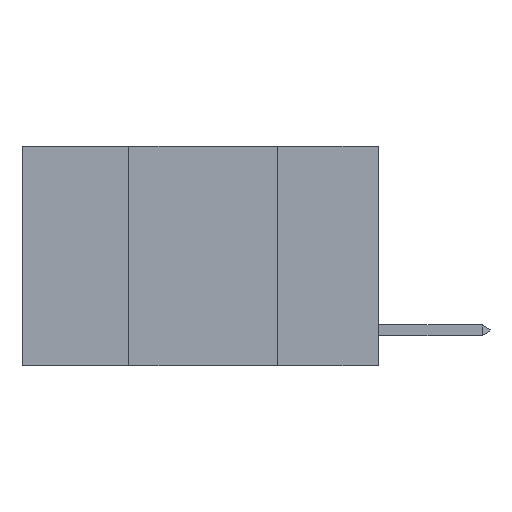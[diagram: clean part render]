
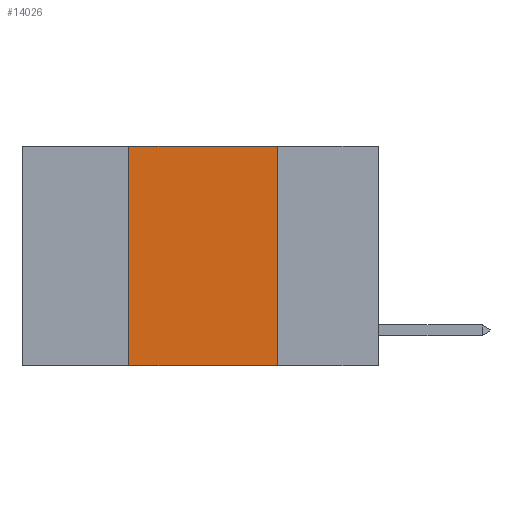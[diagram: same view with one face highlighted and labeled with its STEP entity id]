
A CAD part, left-side view. The second image highlights one B-rep face of the part: STEP entity #14026.
In plain terms, the highlighted planar face has unit normal (-1, 0, 0).
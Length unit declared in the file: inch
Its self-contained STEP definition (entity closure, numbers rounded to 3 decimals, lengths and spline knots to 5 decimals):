
#157 = CARTESIAN_POINT ( 'NONE',  ( 0., 0.42, 0. ) ) ;
#608 = VERTEX_POINT ( 'NONE', #15017 ) ;
#1483 = EDGE_CURVE ( 'NONE', #13183, #608, #8856, .T. ) ;
#1678 = LINE ( 'NONE', #9619, #2033 ) ;
#1892 = VECTOR ( 'NONE', #8744, 39.37008 ) ;
#2033 = VECTOR ( 'NONE', #13283, 39.37008 ) ;
#2262 = LINE ( 'NONE', #9301, #11561 ) ;
#2625 = VERTEX_POINT ( 'NONE', #10244 ) ;
#3862 = EDGE_CURVE ( 'NONE', #608, #2625, #1678, .T. ) ;
#3880 = DIRECTION ( 'NONE',  ( 1., 0., 0. ) ) ;
#4150 = CARTESIAN_POINT ( 'NONE',  ( 0., 0.42, -0.37 ) ) ;
#6782 = CARTESIAN_POINT ( 'NONE',  ( 0., 0.42, 0. ) ) ;
#7122 = ORIENTED_EDGE ( 'NONE', *, *, #15052, .F. ) ;
#8417 = CARTESIAN_POINT ( 'NONE',  ( 0., 0.6, 0. ) ) ;
#8744 = DIRECTION ( 'NONE',  ( 0., 0., 1. ) ) ;
#8856 = LINE ( 'NONE', #8417, #14855 ) ;
#8930 = ORIENTED_EDGE ( 'NONE', *, *, #1483, .F. ) ;
#9301 = CARTESIAN_POINT ( 'NONE',  ( 0., 0.6, -0.37 ) ) ;
#9494 = ORIENTED_EDGE ( 'NONE', *, *, #3862, .F. ) ;
#9543 = EDGE_LOOP ( 'NONE', ( #9494, #8930, #7122, #14382 ) ) ;
#9619 = CARTESIAN_POINT ( 'NONE',  ( 0., 0.17, 0. ) ) ;
#10244 = CARTESIAN_POINT ( 'NONE',  ( 0., 0.17, -0.37 ) ) ;
#11355 = DIRECTION ( 'NONE',  ( 0., -1., 0. ) ) ;
#11404 = FACE_OUTER_BOUND ( 'NONE', #9543, .T. ) ;
#11561 = VECTOR ( 'NONE', #12902, 39.37008 ) ;
#12109 = LINE ( 'NONE', #157, #1892 ) ;
#12122 = VERTEX_POINT ( 'NONE', #4150 ) ;
#12156 = AXIS2_PLACEMENT_3D ( 'NONE', #13621, #3880, #12330 ) ;
#12330 = DIRECTION ( 'NONE',  ( 0., 0., -1. ) ) ;
#12541 = PLANE ( 'NONE',  #12156 ) ;
#12902 = DIRECTION ( 'NONE',  ( 0., -1., 0. ) ) ;
#13183 = VERTEX_POINT ( 'NONE', #6782 ) ;
#13283 = DIRECTION ( 'NONE',  ( 0., 0., -1. ) ) ;
#13621 = CARTESIAN_POINT ( 'NONE',  ( 0., 0.6, 0. ) ) ;
#14026 = ADVANCED_FACE ( 'NONE', ( #11404 ), #12541, .F. ) ;
#14382 = ORIENTED_EDGE ( 'NONE', *, *, #14980, .T. ) ;
#14855 = VECTOR ( 'NONE', #11355, 39.37008 ) ;
#14980 = EDGE_CURVE ( 'NONE', #12122, #2625, #2262, .T. ) ;
#15017 = CARTESIAN_POINT ( 'NONE',  ( 0., 0.17, 0. ) ) ;
#15052 = EDGE_CURVE ( 'NONE', #12122, #13183, #12109, .T. ) ;
